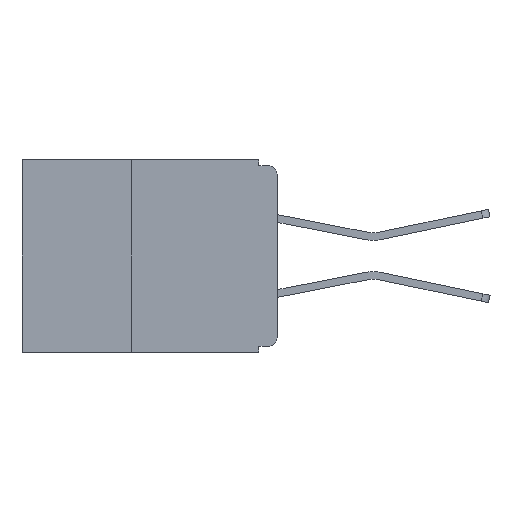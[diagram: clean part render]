
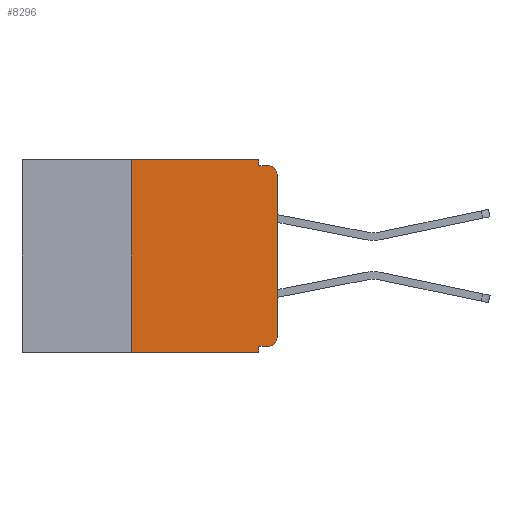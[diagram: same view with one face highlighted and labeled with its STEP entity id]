
A CAD part, left-side view. The second image highlights one B-rep face of the part: STEP entity #8296.
In plain terms, the highlighted planar face has unit normal (-1, 0, 0).
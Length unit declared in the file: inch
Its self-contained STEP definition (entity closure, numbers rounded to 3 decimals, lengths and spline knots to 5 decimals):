
#59 = DIRECTION ( 'NONE',  ( 0., 0., -1. ) ) ;
#119 = ORIENTED_EDGE ( 'NONE', *, *, #2390, .T. ) ;
#127 = CARTESIAN_POINT ( 'NONE',  ( 0., 0.031, -0.33 ) ) ;
#357 = LINE ( 'NONE', #17252, #3630 ) ;
#421 = ORIENTED_EDGE ( 'NONE', *, *, #6805, .F. ) ;
#549 = CARTESIAN_POINT ( 'NONE',  ( 0., 0.015, -0.32 ) ) ;
#666 = CARTESIAN_POINT ( 'NONE',  ( 0., 0.031, -0.33 ) ) ;
#691 = CARTESIAN_POINT ( 'NONE',  ( 0., 0.25, -0.33 ) ) ;
#694 = VECTOR ( 'NONE', #1835, 39.37008 ) ;
#968 = VERTEX_POINT ( 'NONE', #549 ) ;
#1418 = CARTESIAN_POINT ( 'NONE',  ( 0., 0., -0.32 ) ) ;
#1521 = VERTEX_POINT ( 'NONE', #10217 ) ;
#1641 = VERTEX_POINT ( 'NONE', #9154 ) ;
#1835 = DIRECTION ( 'NONE',  ( 0., 0., 1. ) ) ;
#2027 = ORIENTED_EDGE ( 'NONE', *, *, #7231, .T. ) ;
#2271 = CARTESIAN_POINT ( 'NONE',  ( 0., 0.437, -0.33 ) ) ;
#2319 = LINE ( 'NONE', #2271, #9217 ) ;
#2344 = CARTESIAN_POINT ( 'NONE',  ( 0., 0.031, 0. ) ) ;
#2346 = DIRECTION ( 'NONE',  ( 0., 0., -1. ) ) ;
#2390 = EDGE_CURVE ( 'NONE', #15023, #15210, #2684, .T. ) ;
#2555 = ORIENTED_EDGE ( 'NONE', *, *, #10113, .F. ) ;
#2684 = CIRCLE ( 'NONE', #8148, 0.015 ) ;
#2840 = DIRECTION ( 'NONE',  ( 0., 1., 0. ) ) ;
#3292 = DIRECTION ( 'NONE',  ( 1., 0., 0. ) ) ;
#3521 = CIRCLE ( 'NONE', #13136, 0.015 ) ;
#3630 = VECTOR ( 'NONE', #6450, 39.37008 ) ;
#3688 = DIRECTION ( 'NONE',  ( 0., -1., 0. ) ) ;
#3754 = CARTESIAN_POINT ( 'NONE',  ( 0., 0., -0.025 ) ) ;
#3806 = EDGE_CURVE ( 'NONE', #1641, #8712, #7593, .T. ) ;
#4728 = VECTOR ( 'NONE', #2840, 39.37008 ) ;
#4935 = ORIENTED_EDGE ( 'NONE', *, *, #3806, .F. ) ;
#5659 = AXIS2_PLACEMENT_3D ( 'NONE', #8742, #3292, #12831 ) ;
#6450 = DIRECTION ( 'NONE',  ( 0., -1., 0. ) ) ;
#6483 = CARTESIAN_POINT ( 'NONE',  ( 0., 0.015, -0.305 ) ) ;
#6744 = VERTEX_POINT ( 'NONE', #666 ) ;
#6801 = VECTOR ( 'NONE', #9474, 39.37008 ) ;
#6805 = EDGE_CURVE ( 'NONE', #14599, #6744, #8350, .T. ) ;
#7231 = EDGE_CURVE ( 'NONE', #1521, #15023, #15567, .T. ) ;
#7340 = ORIENTED_EDGE ( 'NONE', *, *, #15526, .F. ) ;
#7593 = LINE ( 'NONE', #2344, #11204 ) ;
#7666 = LINE ( 'NONE', #14936, #6801 ) ;
#7848 = DIRECTION ( 'NONE',  ( 0., 0., -1. ) ) ;
#8029 = EDGE_CURVE ( 'NONE', #12785, #1641, #7666, .T. ) ;
#8148 = AXIS2_PLACEMENT_3D ( 'NONE', #16804, #16703, #16441 ) ;
#8248 = CARTESIAN_POINT ( 'NONE',  ( 0., 0.031, -0.32 ) ) ;
#8296 = ADVANCED_FACE ( 'NONE', ( #13814 ), #12778, .F. ) ;
#8334 = VECTOR ( 'NONE', #17142, 39.37008 ) ;
#8350 = LINE ( 'NONE', #127, #15585 ) ;
#8431 = CARTESIAN_POINT ( 'NONE',  ( 0., 0.25, 0. ) ) ;
#8712 = VERTEX_POINT ( 'NONE', #12276 ) ;
#8742 = CARTESIAN_POINT ( 'NONE',  ( 0., 0.437, 0. ) ) ;
#9154 = CARTESIAN_POINT ( 'NONE',  ( 0., 0.031, 0. ) ) ;
#9217 = VECTOR ( 'NONE', #3688, 39.37008 ) ;
#9269 = ORIENTED_EDGE ( 'NONE', *, *, #15473, .T. ) ;
#9474 = DIRECTION ( 'NONE',  ( 0., -1., 0. ) ) ;
#9701 = VERTEX_POINT ( 'NONE', #691 ) ;
#9874 = EDGE_LOOP ( 'NONE', ( #2027, #119, #13111, #4935, #13472, #2555, #9269, #421, #7340, #12730 ) ) ;
#10113 = EDGE_CURVE ( 'NONE', #9701, #12785, #12473, .T. ) ;
#10217 = CARTESIAN_POINT ( 'NONE',  ( 0., 0., -0.305 ) ) ;
#11204 = VECTOR ( 'NONE', #2346, 39.37008 ) ;
#11746 = CARTESIAN_POINT ( 'NONE',  ( 0., 0., 0. ) ) ;
#12256 = EDGE_CURVE ( 'NONE', #968, #1521, #3521, .T. ) ;
#12276 = CARTESIAN_POINT ( 'NONE',  ( 0., 0.031, -0.01 ) ) ;
#12473 = LINE ( 'NONE', #15477, #694 ) ;
#12730 = ORIENTED_EDGE ( 'NONE', *, *, #12256, .T. ) ;
#12778 = PLANE ( 'NONE',  #5659 ) ;
#12785 = VERTEX_POINT ( 'NONE', #8431 ) ;
#12831 = DIRECTION ( 'NONE',  ( 0., 0., -1. ) ) ;
#13111 = ORIENTED_EDGE ( 'NONE', *, *, #15833, .F. ) ;
#13136 = AXIS2_PLACEMENT_3D ( 'NONE', #6483, #15994, #7848 ) ;
#13472 = ORIENTED_EDGE ( 'NONE', *, *, #8029, .F. ) ;
#13814 = FACE_OUTER_BOUND ( 'NONE', #9874, .T. ) ;
#14599 = VERTEX_POINT ( 'NONE', #8248 ) ;
#14936 = CARTESIAN_POINT ( 'NONE',  ( 0., 0.437, 0. ) ) ;
#15023 = VERTEX_POINT ( 'NONE', #3754 ) ;
#15210 = VERTEX_POINT ( 'NONE', #16664 ) ;
#15473 = EDGE_CURVE ( 'NONE', #9701, #6744, #2319, .T. ) ;
#15477 = CARTESIAN_POINT ( 'NONE',  ( 0., 0.25, -0.33 ) ) ;
#15526 = EDGE_CURVE ( 'NONE', #968, #14599, #15574, .T. ) ;
#15567 = LINE ( 'NONE', #11746, #8334 ) ;
#15574 = LINE ( 'NONE', #1418, #4728 ) ;
#15585 = VECTOR ( 'NONE', #59, 39.37008 ) ;
#15833 = EDGE_CURVE ( 'NONE', #8712, #15210, #357, .T. ) ;
#15994 = DIRECTION ( 'NONE',  ( -1., 0., 0. ) ) ;
#16441 = DIRECTION ( 'NONE',  ( 0., 0., -1. ) ) ;
#16664 = CARTESIAN_POINT ( 'NONE',  ( 0., 0.015, -0.01 ) ) ;
#16703 = DIRECTION ( 'NONE',  ( -1., 0., 0. ) ) ;
#16804 = CARTESIAN_POINT ( 'NONE',  ( 0., 0.015, -0.025 ) ) ;
#17142 = DIRECTION ( 'NONE',  ( 0., 0., 1. ) ) ;
#17252 = CARTESIAN_POINT ( 'NONE',  ( 0., 0., -0.01 ) ) ;
